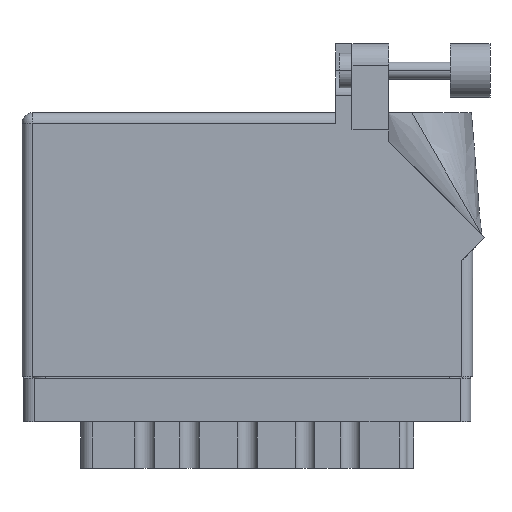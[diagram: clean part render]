
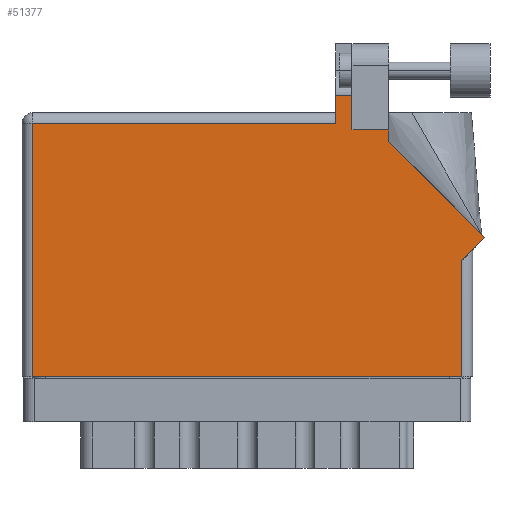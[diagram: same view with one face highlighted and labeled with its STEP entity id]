
A CAD part, front view. The second image highlights one B-rep face of the part: STEP entity #51377.
In plain terms, the highlighted face is planar.
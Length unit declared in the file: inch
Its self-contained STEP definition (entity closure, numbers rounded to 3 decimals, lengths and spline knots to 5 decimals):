
#123 = LINE ( 'NONE', #18202, #26184 ) ;
#1179 = VERTEX_POINT ( 'NONE', #24223 ) ;
#1274 = ORIENTED_EDGE ( 'NONE', *, *, #51789, .T. ) ;
#1674 = DIRECTION ( 'NONE',  ( -0.707, 0.707, 0. ) ) ;
#1890 = CARTESIAN_POINT ( 'NONE',  ( 0.062, 0., 0. ) ) ;
#2788 = DIRECTION ( 'NONE',  ( -1., 0., 0. ) ) ;
#2825 = VERTEX_POINT ( 'NONE', #35782 ) ;
#2991 = ORIENTED_EDGE ( 'NONE', *, *, #33964, .T. ) ;
#5015 = EDGE_CURVE ( 'NONE', #2825, #1179, #21964, .T. ) ;
#5021 = DIRECTION ( 'NONE',  ( 0., 1., 0. ) ) ;
#5090 = EDGE_CURVE ( 'NONE', #24092, #51493, #40201, .T. ) ;
#5102 = ORIENTED_EDGE ( 'NONE', *, *, #43099, .T. ) ;
#6966 = VECTOR ( 'NONE', #49387, 39.37008 ) ;
#7627 = FACE_OUTER_BOUND ( 'NONE', #8800, .T. ) ;
#7818 = VECTOR ( 'NONE', #20256, 39.37008 ) ;
#8800 = EDGE_LOOP ( 'NONE', ( #39831, #1274, #39872, #20693, #32803, #2991, #21738, #53978, #16541, #16490, #5102 ) ) ;
#9291 = VECTOR ( 'NONE', #5021, 39.37008 ) ;
#9359 = CARTESIAN_POINT ( 'NONE',  ( 2.55, 0.737, 0. ) ) ;
#10623 = DIRECTION ( 'NONE',  ( 0., -1., 0. ) ) ;
#10725 = LINE ( 'NONE', #25513, #45309 ) ;
#10821 = DIRECTION ( 'NONE',  ( 1., 0., 0. ) ) ;
#11853 = CARTESIAN_POINT ( 'NONE',  ( 2.24377, 1.6315, 0. ) ) ;
#14077 = LINE ( 'NONE', #1890, #22574 ) ;
#14303 = VECTOR ( 'NONE', #50967, 39.37008 ) ;
#14781 = VECTOR ( 'NONE', #35887, 39.37008 ) ;
#16279 = LINE ( 'NONE', #11853, #7818 ) ;
#16490 = ORIENTED_EDGE ( 'NONE', *, *, #48020, .T. ) ;
#16541 = ORIENTED_EDGE ( 'NONE', *, *, #38931, .T. ) ;
#17110 = LINE ( 'NONE', #25075, #9291 ) ;
#18202 = CARTESIAN_POINT ( 'NONE',  ( 2.68271, 0.80771, 0. ) ) ;
#18750 = CARTESIAN_POINT ( 'NONE',  ( 1.819, 1.53, 0. ) ) ;
#19553 = VERTEX_POINT ( 'NONE', #34783 ) ;
#20256 = DIRECTION ( 'NONE',  ( -1., 0., 0. ) ) ;
#20631 = VECTOR ( 'NONE', #10821, 39.37008 ) ;
#20693 = ORIENTED_EDGE ( 'NONE', *, *, #42842, .T. ) ;
#20960 = EDGE_CURVE ( 'NONE', #22195, #48250, #14077, .T. ) ;
#21738 = ORIENTED_EDGE ( 'NONE', *, *, #40464, .T. ) ;
#21887 = AXIS2_PLACEMENT_3D ( 'NONE', #42127, #50226, #46741 ) ;
#21964 = LINE ( 'NONE', #18750, #14781 ) ;
#22075 = LINE ( 'NONE', #28909, #42346 ) ;
#22195 = VERTEX_POINT ( 'NONE', #22697 ) ;
#22574 = VECTOR ( 'NONE', #10623, 39.37008 ) ;
#22697 = CARTESIAN_POINT ( 'NONE',  ( 0.062, 1.468, 0. ) ) ;
#23551 = CARTESIAN_POINT ( 'NONE',  ( 0., 1.468, 0. ) ) ;
#23830 = CARTESIAN_POINT ( 'NONE',  ( 2.612, 0.737, 0. ) ) ;
#23949 = CARTESIAN_POINT ( 'NONE',  ( 2.55, 0., 0. ) ) ;
#24092 = VERTEX_POINT ( 'NONE', #46644 ) ;
#24223 = CARTESIAN_POINT ( 'NONE',  ( 1.819, 1.468, 0. ) ) ;
#25075 = CARTESIAN_POINT ( 'NONE',  ( 2.126, 1.36442, 0. ) ) ;
#25513 = CARTESIAN_POINT ( 'NONE',  ( 2.126, 1.43, 0. ) ) ;
#25680 = CARTESIAN_POINT ( 'NONE',  ( 2.126, 1.43, 0. ) ) ;
#26184 = VECTOR ( 'NONE', #1674, 39.37008 ) ;
#28019 = LINE ( 'NONE', #9359, #14303 ) ;
#28909 = CARTESIAN_POINT ( 'NONE',  ( 1.913, 1.43, 0. ) ) ;
#29792 = VERTEX_POINT ( 'NONE', #23949 ) ;
#30669 = VERTEX_POINT ( 'NONE', #25680 ) ;
#31594 = CARTESIAN_POINT ( 'NONE',  ( 0., 0., 0. ) ) ;
#31631 = EDGE_CURVE ( 'NONE', #53389, #19553, #22075, .T. ) ;
#32803 = ORIENTED_EDGE ( 'NONE', *, *, #20960, .T. ) ;
#32993 = LINE ( 'NONE', #31594, #20631 ) ;
#33158 = DIRECTION ( 'NONE',  ( -1., 0., 0. ) ) ;
#33278 = DIRECTION ( 'NONE',  ( 0., 1., 0. ) ) ;
#33964 = EDGE_CURVE ( 'NONE', #48250, #29792, #32993, .T. ) ;
#34783 = CARTESIAN_POINT ( 'NONE',  ( 1.913, 1.6315, 0. ) ) ;
#35782 = CARTESIAN_POINT ( 'NONE',  ( 1.819, 1.6315, 0. ) ) ;
#35887 = DIRECTION ( 'NONE',  ( 0., -1., 0. ) ) ;
#36759 = CARTESIAN_POINT ( 'NONE',  ( 1.913, 1.43, 0. ) ) ;
#38931 = EDGE_CURVE ( 'NONE', #51493, #50629, #123, .T. ) ;
#39191 = CARTESIAN_POINT ( 'NONE',  ( 2.68271, 0.80771, 0. ) ) ;
#39831 = ORIENTED_EDGE ( 'NONE', *, *, #31631, .T. ) ;
#39872 = ORIENTED_EDGE ( 'NONE', *, *, #5015, .T. ) ;
#40101 = VECTOR ( 'NONE', #2788, 39.37008 ) ;
#40201 = LINE ( 'NONE', #23830, #6966 ) ;
#40464 = EDGE_CURVE ( 'NONE', #29792, #24092, #28019, .T. ) ;
#42079 = LINE ( 'NONE', #23551, #40101 ) ;
#42127 = CARTESIAN_POINT ( 'NONE',  ( 0., 1.53, 0. ) ) ;
#42346 = VECTOR ( 'NONE', #33278, 39.37008 ) ;
#42842 = EDGE_CURVE ( 'NONE', #1179, #22195, #42079, .T. ) ;
#43099 = EDGE_CURVE ( 'NONE', #30669, #53389, #10725, .T. ) ;
#43452 = CARTESIAN_POINT ( 'NONE',  ( 0.062, 0., 0. ) ) ;
#45309 = VECTOR ( 'NONE', #33158, 39.37008 ) ;
#45709 = CARTESIAN_POINT ( 'NONE',  ( 2.126, 1.36442, 0. ) ) ;
#46644 = CARTESIAN_POINT ( 'NONE',  ( 2.55, 0.675, 0. ) ) ;
#46741 = DIRECTION ( 'NONE',  ( -1., 0., 0. ) ) ;
#48020 = EDGE_CURVE ( 'NONE', #50629, #30669, #17110, .T. ) ;
#48250 = VERTEX_POINT ( 'NONE', #43452 ) ;
#49387 = DIRECTION ( 'NONE',  ( 0.707, 0.707, 0. ) ) ;
#50226 = DIRECTION ( 'NONE',  ( 0., 0., -1. ) ) ;
#50408 = PLANE ( 'NONE',  #21887 ) ;
#50629 = VERTEX_POINT ( 'NONE', #45709 ) ;
#50967 = DIRECTION ( 'NONE',  ( 0., 1., 0. ) ) ;
#51377 = ADVANCED_FACE ( 'NONE', ( #7627 ), #50408, .F. ) ;
#51493 = VERTEX_POINT ( 'NONE', #39191 ) ;
#51789 = EDGE_CURVE ( 'NONE', #19553, #2825, #16279, .T. ) ;
#53389 = VERTEX_POINT ( 'NONE', #36759 ) ;
#53978 = ORIENTED_EDGE ( 'NONE', *, *, #5090, .T. ) ;
